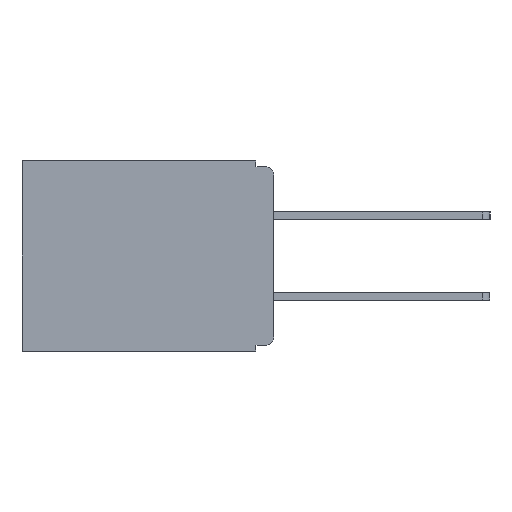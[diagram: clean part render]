
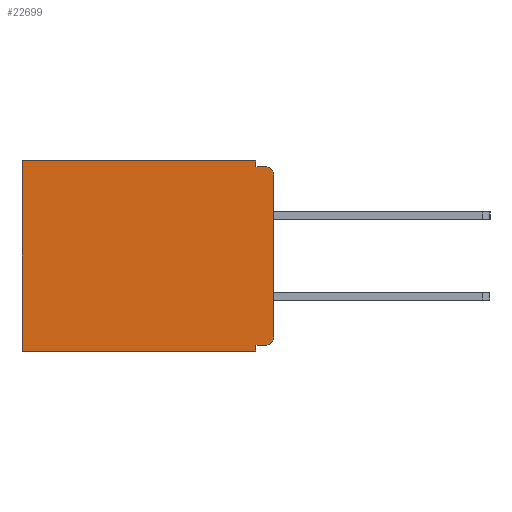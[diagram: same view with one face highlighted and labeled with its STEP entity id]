
A CAD part, left-side view. The second image highlights one B-rep face of the part: STEP entity #22699.
In plain terms, the highlighted planar face has unit normal (-1, 0, 0).
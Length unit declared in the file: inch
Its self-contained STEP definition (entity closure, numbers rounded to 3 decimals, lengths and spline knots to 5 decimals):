
#232 = VECTOR ( 'NONE', #2618, 39.37008 ) ;
#976 = LINE ( 'NONE', #26097, #12893 ) ;
#1233 = CARTESIAN_POINT ( 'NONE',  ( 0.3, 0.015, -0.32 ) ) ;
#1325 = VERTEX_POINT ( 'NONE', #16953 ) ;
#1386 = EDGE_CURVE ( 'NONE', #28756, #23194, #976, .T. ) ;
#1446 = VECTOR ( 'NONE', #3972, 39.37008 ) ;
#2128 = LINE ( 'NONE', #24128, #1446 ) ;
#2618 = DIRECTION ( 'NONE',  ( 0., 1., 0. ) ) ;
#2642 = CARTESIAN_POINT ( 'NONE',  ( 0.3, 0., -0.33 ) ) ;
#3004 = LINE ( 'NONE', #15797, #20206 ) ;
#3042 = ORIENTED_EDGE ( 'NONE', *, *, #14620, .T. ) ;
#3131 = CARTESIAN_POINT ( 'NONE',  ( 0.3, 0.015, -0.01 ) ) ;
#3527 = VERTEX_POINT ( 'NONE', #25448 ) ;
#3972 = DIRECTION ( 'NONE',  ( 0., 1., 0. ) ) ;
#4009 = CARTESIAN_POINT ( 'NONE',  ( 0.3, 0.437, 0. ) ) ;
#4087 = VECTOR ( 'NONE', #24505, 39.37008 ) ;
#4246 = VERTEX_POINT ( 'NONE', #27492 ) ;
#4542 = CARTESIAN_POINT ( 'NONE',  ( 0.3, 0., -0.32 ) ) ;
#5147 = AXIS2_PLACEMENT_3D ( 'NONE', #26215, #12726, #28414 ) ;
#5675 = FACE_OUTER_BOUND ( 'NONE', #17180, .T. ) ;
#5816 = VERTEX_POINT ( 'NONE', #24048 ) ;
#6498 = CARTESIAN_POINT ( 'NONE',  ( 0.3, 0.031, 0. ) ) ;
#6508 = CARTESIAN_POINT ( 'NONE',  ( 0.3, 0.031, -0.01 ) ) ;
#6898 = ORIENTED_EDGE ( 'NONE', *, *, #23794, .F. ) ;
#7620 = ORIENTED_EDGE ( 'NONE', *, *, #17589, .F. ) ;
#7984 = EDGE_CURVE ( 'NONE', #4246, #5816, #26034, .T. ) ;
#8605 = CARTESIAN_POINT ( 'NONE',  ( 0.3, 0.437, -0.33 ) ) ;
#8714 = EDGE_CURVE ( 'NONE', #26504, #3527, #13663, .T. ) ;
#8985 = DIRECTION ( 'NONE',  ( 0., -1., 0. ) ) ;
#9115 = CARTESIAN_POINT ( 'NONE',  ( 0.3, 0., -0.33 ) ) ;
#10035 = EDGE_CURVE ( 'NONE', #20166, #5816, #18128, .T. ) ;
#10214 = EDGE_CURVE ( 'NONE', #1325, #20508, #26616, .T. ) ;
#11171 = AXIS2_PLACEMENT_3D ( 'NONE', #9115, #24867, #11368 ) ;
#11277 = PLANE ( 'NONE',  #11171 ) ;
#11368 = DIRECTION ( 'NONE',  ( 0., 0., -1. ) ) ;
#11623 = CARTESIAN_POINT ( 'NONE',  ( 0.3, 0.031, -0.33 ) ) ;
#11883 = CIRCLE ( 'NONE', #22386, 0.015 ) ;
#12129 = LINE ( 'NONE', #22744, #232 ) ;
#12202 = ORIENTED_EDGE ( 'NONE', *, *, #8714, .F. ) ;
#12343 = VECTOR ( 'NONE', #13610, 39.37008 ) ;
#12726 = DIRECTION ( 'NONE',  ( -1., 0., 0. ) ) ;
#12749 = CARTESIAN_POINT ( 'NONE',  ( 0.3, 0.015, -0.025 ) ) ;
#12893 = VECTOR ( 'NONE', #25758, 39.37008 ) ;
#12958 = VECTOR ( 'NONE', #22738, 39.37008 ) ;
#13054 = LINE ( 'NONE', #4542, #12343 ) ;
#13261 = ORIENTED_EDGE ( 'NONE', *, *, #10214, .F. ) ;
#13610 = DIRECTION ( 'NONE',  ( 0., 1., 0. ) ) ;
#13663 = LINE ( 'NONE', #11623, #12958 ) ;
#14620 = EDGE_CURVE ( 'NONE', #4246, #27748, #11883, .T. ) ;
#14793 = VECTOR ( 'NONE', #18354, 39.37008 ) ;
#15045 = DIRECTION ( 'NONE',  ( 0., 0., -1. ) ) ;
#15057 = ORIENTED_EDGE ( 'NONE', *, *, #10035, .T. ) ;
#15797 = CARTESIAN_POINT ( 'NONE',  ( 0.3, 0., -0.01 ) ) ;
#16087 = ORIENTED_EDGE ( 'NONE', *, *, #26663, .F. ) ;
#16953 = CARTESIAN_POINT ( 'NONE',  ( 0.3, 0.031, 0. ) ) ;
#17134 = ORIENTED_EDGE ( 'NONE', *, *, #7984, .F. ) ;
#17180 = EDGE_LOOP ( 'NONE', ( #17134, #3042, #16087, #13261, #17492, #28019, #6898, #12202, #7620, #15057 ) ) ;
#17492 = ORIENTED_EDGE ( 'NONE', *, *, #26754, .T. ) ;
#17589 = EDGE_CURVE ( 'NONE', #20166, #26504, #13054, .T. ) ;
#18128 = CIRCLE ( 'NONE', #5147, 0.015 ) ;
#18354 = DIRECTION ( 'NONE',  ( 0., 0., -1. ) ) ;
#20166 = VERTEX_POINT ( 'NONE', #1233 ) ;
#20206 = VECTOR ( 'NONE', #8985, 39.37008 ) ;
#20508 = VERTEX_POINT ( 'NONE', #6508 ) ;
#22386 = AXIS2_PLACEMENT_3D ( 'NONE', #12749, #28438, #15045 ) ;
#22699 = ADVANCED_FACE ( 'NONE', ( #5675 ), #11277, .F. ) ;
#22738 = DIRECTION ( 'NONE',  ( 0., 0., -1. ) ) ;
#22744 = CARTESIAN_POINT ( 'NONE',  ( 0.3, 0., 0. ) ) ;
#23194 = VERTEX_POINT ( 'NONE', #8605 ) ;
#23794 = EDGE_CURVE ( 'NONE', #3527, #23194, #2128, .T. ) ;
#24048 = CARTESIAN_POINT ( 'NONE',  ( 0.3, 0., -0.305 ) ) ;
#24128 = CARTESIAN_POINT ( 'NONE',  ( 0.3, 0., -0.33 ) ) ;
#24505 = DIRECTION ( 'NONE',  ( 0., 0., -1. ) ) ;
#24867 = DIRECTION ( 'NONE',  ( 1., 0., 0. ) ) ;
#25448 = CARTESIAN_POINT ( 'NONE',  ( 0.3, 0.031, -0.33 ) ) ;
#25758 = DIRECTION ( 'NONE',  ( 0., 0., -1. ) ) ;
#26034 = LINE ( 'NONE', #2642, #14793 ) ;
#26097 = CARTESIAN_POINT ( 'NONE',  ( 0.3, 0.437, -0.33 ) ) ;
#26215 = CARTESIAN_POINT ( 'NONE',  ( 0.3, 0.015, -0.305 ) ) ;
#26436 = CARTESIAN_POINT ( 'NONE',  ( 0.3, 0.031, -0.32 ) ) ;
#26504 = VERTEX_POINT ( 'NONE', #26436 ) ;
#26616 = LINE ( 'NONE', #6498, #4087 ) ;
#26663 = EDGE_CURVE ( 'NONE', #20508, #27748, #3004, .T. ) ;
#26754 = EDGE_CURVE ( 'NONE', #1325, #28756, #12129, .T. ) ;
#27492 = CARTESIAN_POINT ( 'NONE',  ( 0.3, 0., -0.025 ) ) ;
#27748 = VERTEX_POINT ( 'NONE', #3131 ) ;
#28019 = ORIENTED_EDGE ( 'NONE', *, *, #1386, .T. ) ;
#28414 = DIRECTION ( 'NONE',  ( 0., 0., -1. ) ) ;
#28438 = DIRECTION ( 'NONE',  ( -1., 0., 0. ) ) ;
#28756 = VERTEX_POINT ( 'NONE', #4009 ) ;
